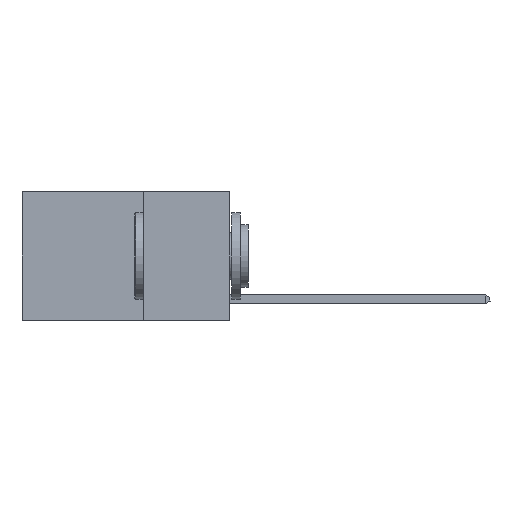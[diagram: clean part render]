
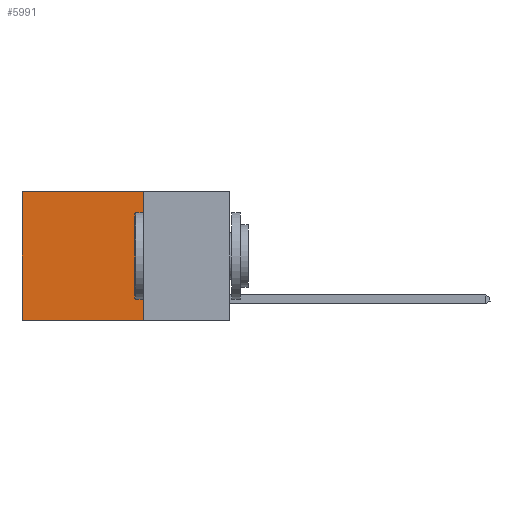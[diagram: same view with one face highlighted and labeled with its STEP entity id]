
A CAD part, left-side view. The second image highlights one B-rep face of the part: STEP entity #5991.
In plain terms, the highlighted planar face has unit normal (-1, 0, 0).
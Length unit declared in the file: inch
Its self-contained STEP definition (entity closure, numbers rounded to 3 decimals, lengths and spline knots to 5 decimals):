
#71 = CARTESIAN_POINT ( 'NONE',  ( 0.2625, 0.25, 0. ) ) ;
#1208 = CARTESIAN_POINT ( 'NONE',  ( 0.2625, 0.6, -0.37 ) ) ;
#2787 = FACE_OUTER_BOUND ( 'NONE', #26010, .T. ) ;
#3313 = DIRECTION ( 'NONE',  ( 0., 1., 0. ) ) ;
#4436 = VECTOR ( 'NONE', #13739, 39.37008 ) ;
#4665 = DIRECTION ( 'NONE',  ( 1., 0., 0. ) ) ;
#4953 = EDGE_CURVE ( 'NONE', #23942, #26402, #21732, .T. ) ;
#5439 = CARTESIAN_POINT ( 'NONE',  ( 0.2625, 0.25, -0.37 ) ) ;
#5991 = ADVANCED_FACE ( 'NONE', ( #2787 ), #11565, .F. ) ;
#6096 = LINE ( 'NONE', #13997, #17788 ) ;
#6828 = ORIENTED_EDGE ( 'NONE', *, *, #26099, .T. ) ;
#7649 = VECTOR ( 'NONE', #21048, 39.37008 ) ;
#10101 = ORIENTED_EDGE ( 'NONE', *, *, #24710, .F. ) ;
#10594 = LINE ( 'NONE', #29961, #4436 ) ;
#11565 = PLANE ( 'NONE',  #29684 ) ;
#12526 = CARTESIAN_POINT ( 'NONE',  ( 0.2625, 0.25, -0.37 ) ) ;
#13557 = ORIENTED_EDGE ( 'NONE', *, *, #21166, .T. ) ;
#13739 = DIRECTION ( 'NONE',  ( 0., 1., 0. ) ) ;
#13816 = LINE ( 'NONE', #71, #7649 ) ;
#13899 = DIRECTION ( 'NONE',  ( 0., 0., -1. ) ) ;
#13997 = CARTESIAN_POINT ( 'NONE',  ( 0.2625, 0.6, 0. ) ) ;
#15491 = VECTOR ( 'NONE', #3313, 39.37008 ) ;
#15492 = VERTEX_POINT ( 'NONE', #24148 ) ;
#16447 = VERTEX_POINT ( 'NONE', #25507 ) ;
#17788 = VECTOR ( 'NONE', #13899, 39.37008 ) ;
#18622 = CARTESIAN_POINT ( 'NONE',  ( 0.2625, 0.25, 0. ) ) ;
#20984 = DIRECTION ( 'NONE',  ( 0., 0., -1. ) ) ;
#21048 = DIRECTION ( 'NONE',  ( 0., 0., -1. ) ) ;
#21166 = EDGE_CURVE ( 'NONE', #16447, #15492, #10594, .T. ) ;
#21732 = LINE ( 'NONE', #12526, #15491 ) ;
#22052 = ORIENTED_EDGE ( 'NONE', *, *, #4953, .F. ) ;
#23942 = VERTEX_POINT ( 'NONE', #5439 ) ;
#24148 = CARTESIAN_POINT ( 'NONE',  ( 0.2625, 0.6, 0. ) ) ;
#24710 = EDGE_CURVE ( 'NONE', #16447, #23942, #13816, .T. ) ;
#25507 = CARTESIAN_POINT ( 'NONE',  ( 0.2625, 0.25, 0. ) ) ;
#26010 = EDGE_LOOP ( 'NONE', ( #6828, #22052, #10101, #13557 ) ) ;
#26099 = EDGE_CURVE ( 'NONE', #15492, #26402, #6096, .T. ) ;
#26402 = VERTEX_POINT ( 'NONE', #1208 ) ;
#29684 = AXIS2_PLACEMENT_3D ( 'NONE', #18622, #4665, #20984 ) ;
#29961 = CARTESIAN_POINT ( 'NONE',  ( 0.2625, 0.25, 0. ) ) ;
